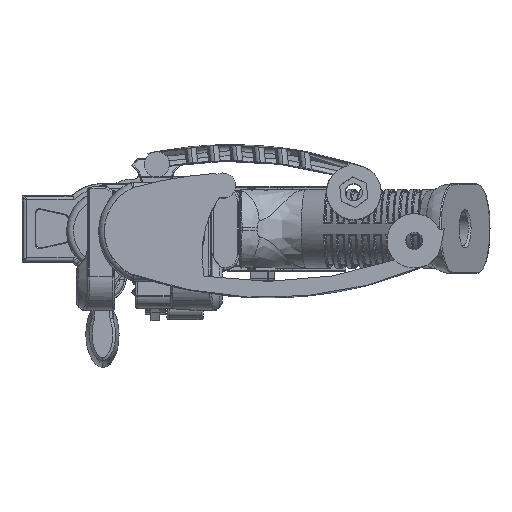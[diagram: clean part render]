
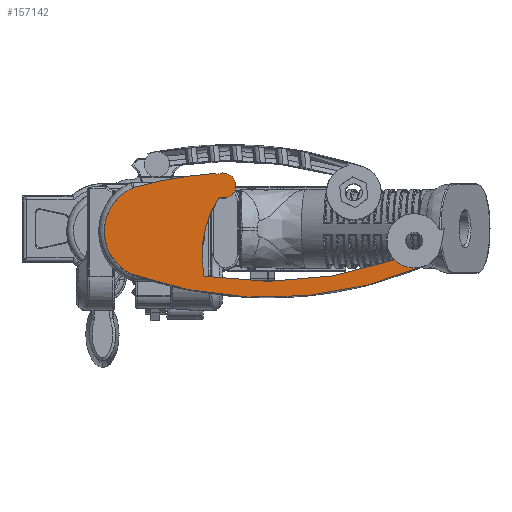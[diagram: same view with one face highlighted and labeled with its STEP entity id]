
A CAD part, left-side view. The second image highlights one B-rep face of the part: STEP entity #157142.
In plain terms, the highlighted face is planar.
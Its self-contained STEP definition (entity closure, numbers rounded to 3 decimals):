
#2163 = VERTEX_POINT ( 'NONE', #118752 ) ;
#6888 = DIRECTION ( 'NONE',  ( 0.225, 0.974, -0.001 ) ) ;
#11616 = PLANE ( 'NONE',  #102818 ) ;
#17375 = CARTESIAN_POINT ( 'NONE',  ( -135.895, 121.89, 0.068 ) ) ;
#17777 = CIRCLE ( 'NONE', #116004, 173.283 ) ;
#17848 = AXIS2_PLACEMENT_3D ( 'NONE', #35511, #21081, #66289 ) ;
#18485 = CARTESIAN_POINT ( 'NONE',  ( -140.622, 167.617, 0.045 ) ) ;
#21081 = DIRECTION ( 'NONE',  ( 0., -0.001, -1. ) ) ;
#22280 = EDGE_CURVE ( 'NONE', #179612, #34762, #17777, .T. ) ;
#25071 = DIRECTION ( 'NONE',  ( -1., -0.017, 0. ) ) ;
#28363 = CIRCLE ( 'NONE', #135728, 12.15 ) ;
#31294 = ORIENTED_EDGE ( 'NONE', *, *, #73756, .T. ) ;
#31754 = CARTESIAN_POINT ( 'NONE',  ( -147.764, 119.293, 0.07 ) ) ;
#34004 = EDGE_CURVE ( 'NONE', #134098, #171112, #118427, .T. ) ;
#34762 = VERTEX_POINT ( 'NONE', #101639 ) ;
#35511 = CARTESIAN_POINT ( 'NONE',  ( -149.801, 236.275, 0.011 ) ) ;
#42200 = VECTOR ( 'NONE', #135635, 1000. ) ;
#43919 = CARTESIAN_POINT ( 'NONE',  ( -171.539, 199.341, 0.031 ) ) ;
#57776 = DIRECTION ( 'NONE',  ( -1., -0.017, 0. ) ) ;
#58803 = EDGE_CURVE ( 'NONE', #2163, #171112, #179771, .T. ) ;
#58984 = ORIENTED_EDGE ( 'NONE', *, *, #189243, .T. ) ;
#66289 = DIRECTION ( 'NONE',  ( -1., -0.017, 0. ) ) ;
#67640 = DIRECTION ( 'NONE',  ( -1., -0.017, 0. ) ) ;
#69297 = CARTESIAN_POINT ( 'NONE',  ( -170.814, 204.868, 0.028 ) ) ;
#70870 = EDGE_CURVE ( 'NONE', #131765, #117530, #28363, .T. ) ;
#71812 = CARTESIAN_POINT ( 'NONE',  ( -301.679, 187.541, 0.048 ) ) ;
#73756 = EDGE_CURVE ( 'NONE', #117530, #179612, #114339, .T. ) ;
#74962 = CARTESIAN_POINT ( 'NONE',  ( -176.143, 208.256, 0.027 ) ) ;
#79977 = DIRECTION ( 'NONE',  ( 0., 0.001, 1. ) ) ;
#80872 = DIRECTION ( 'NONE',  ( 0.988, -0.154, 0. ) ) ;
#82163 = VERTEX_POINT ( 'NONE', #43919 ) ;
#83960 = CARTESIAN_POINT ( 'NONE',  ( -170.814, 204.868, 0.028 ) ) ;
#84330 = DIRECTION ( 'NONE',  ( 0.916, -0.402, 0. ) ) ;
#85887 = EDGE_CURVE ( 'NONE', #34762, #95632, #116286, .T. ) ;
#86778 = CIRCLE ( 'NONE', #123628, 5.574 ) ;
#87002 = ORIENTED_EDGE ( 'NONE', *, *, #34004, .F. ) ;
#89101 = ORIENTED_EDGE ( 'NONE', *, *, #70870, .T. ) ;
#89739 = CARTESIAN_POINT ( 'NONE',  ( -147.764, 119.293, 0.07 ) ) ;
#90517 = CARTESIAN_POINT ( 'NONE',  ( -164.658, 200.954, 0.03 ) ) ;
#95632 = VERTEX_POINT ( 'NONE', #145688 ) ;
#96232 = DIRECTION ( 'NONE',  ( 0., 0.001, 1. ) ) ;
#101639 = CARTESIAN_POINT ( 'NONE',  ( -130.222, 212.629, 0.021 ) ) ;
#102818 = AXIS2_PLACEMENT_3D ( 'NONE', #128842, #96232, #80872 ) ;
#103383 = ORIENTED_EDGE ( 'NONE', *, *, #165769, .T. ) ;
#105563 = AXIS2_PLACEMENT_3D ( 'NONE', #113901, #141787, #110118 ) ;
#110118 = DIRECTION ( 'NONE',  ( 0.947, 0.321, 0. ) ) ;
#112430 = VERTEX_POINT ( 'NONE', #170478 ) ;
#112457 = ORIENTED_EDGE ( 'NONE', *, *, #148379, .T. ) ;
#112848 = DIRECTION ( 'NONE',  ( 0., 0.001, 1. ) ) ;
#113901 = CARTESIAN_POINT ( 'NONE',  ( -301.679, 187.541, 0.048 ) ) ;
#114339 = CIRCLE ( 'NONE', #184909, 12.15 ) ;
#115414 = DIRECTION ( 'NONE',  ( 0., 0.001, 1. ) ) ;
#116004 = AXIS2_PLACEMENT_3D ( 'NONE', #71812, #173586, #84330 ) ;
#116181 = ORIENTED_EDGE ( 'NONE', *, *, #85887, .T. ) ;
#116286 = CIRCLE ( 'NONE', #140843, 46.197 ) ;
#117530 = VERTEX_POINT ( 'NONE', #17375 ) ;
#118427 = CIRCLE ( 'NONE', #146022, 180.483 ) ;
#118752 = CARTESIAN_POINT ( 'NONE',  ( -175.519, 207.859, 0.027 ) ) ;
#123628 = AXIS2_PLACEMENT_3D ( 'NONE', #83960, #127173, #67640 ) ;
#125954 = DIRECTION ( 'NONE',  ( 0., -0.001, -1. ) ) ;
#127173 = DIRECTION ( 'NONE',  ( 0., -0.001, -1. ) ) ;
#128842 = CARTESIAN_POINT ( 'NONE',  ( -149.839, 214.119, 0.022 ) ) ;
#130134 = DIRECTION ( 'NONE',  ( -1., -0.017, 0. ) ) ;
#131765 = VERTEX_POINT ( 'NONE', #178070 ) ;
#134098 = VERTEX_POINT ( 'NONE', #138756 ) ;
#135635 = DIRECTION ( 'NONE',  ( -0.844, 0.536, 0. ) ) ;
#135728 = AXIS2_PLACEMENT_3D ( 'NONE', #89739, #148332, #130134 ) ;
#138756 = CARTESIAN_POINT ( 'NONE',  ( -169.185, 244.736, 0.008 ) ) ;
#138831 = CARTESIAN_POINT ( 'NONE',  ( 3.681, 192.859, 0.021 ) ) ;
#139344 = EDGE_CURVE ( 'NONE', #112430, #131765, #157689, .T. ) ;
#140843 = AXIS2_PLACEMENT_3D ( 'NONE', #18485, #79977, #6888 ) ;
#141787 = DIRECTION ( 'NONE',  ( 0., -0.001, -1. ) ) ;
#144307 = EDGE_LOOP ( 'NONE', ( #87002, #103383, #171432, #89101, #31294, #169860, #116181, #112457, #58984, #158308 ) ) ;
#145688 = CARTESIAN_POINT ( 'NONE',  ( -165.498, 206.545, 0.027 ) ) ;
#146022 = AXIS2_PLACEMENT_3D ( 'NONE', #138831, #112848, #183898 ) ;
#148332 = DIRECTION ( 'NONE',  ( 0., 0.001, 1. ) ) ;
#148379 = EDGE_CURVE ( 'NONE', #95632, #82163, #161626, .T. ) ;
#157142 = ADVANCED_FACE ( 'NONE', ( #187394 ), #11616, .F. ) ;
#157689 = CIRCLE ( 'NONE', #105563, 180.483 ) ;
#158308 = ORIENTED_EDGE ( 'NONE', *, *, #58803, .T. ) ;
#161626 = CIRCLE ( 'NONE', #189286, 5.574 ) ;
#165769 = EDGE_CURVE ( 'NONE', #134098, #112430, #171187, .T. ) ;
#169860 = ORIENTED_EDGE ( 'NONE', *, *, #22280, .T. ) ;
#170478 = CARTESIAN_POINT ( 'NONE',  ( -130.724, 245.406, 0.005 ) ) ;
#171112 = VERTEX_POINT ( 'NONE', #74962 ) ;
#171187 = CIRCLE ( 'NONE', #17848, 21.15 ) ;
#171432 = ORIENTED_EDGE ( 'NONE', *, *, #139344, .T. ) ;
#173586 = DIRECTION ( 'NONE',  ( 0., 0.001, 1. ) ) ;
#176201 = CARTESIAN_POINT ( 'NONE',  ( -139.039, 127.749, 0.065 ) ) ;
#178070 = CARTESIAN_POINT ( 'NONE',  ( -136.305, 115.254, 0.071 ) ) ;
#179612 = VERTEX_POINT ( 'NONE', #176201 ) ;
#179771 = LINE ( 'NONE', #90517, #42200 ) ;
#183898 = DIRECTION ( 'NONE',  ( -0.958, 0.287, 0. ) ) ;
#184909 = AXIS2_PLACEMENT_3D ( 'NONE', #31754, #115414, #57776 ) ;
#187394 = FACE_OUTER_BOUND ( 'NONE', #144307, .T. ) ;
#189243 = EDGE_CURVE ( 'NONE', #82163, #2163, #86778, .T. ) ;
#189286 = AXIS2_PLACEMENT_3D ( 'NONE', #69297, #125954, #25071 ) ;
